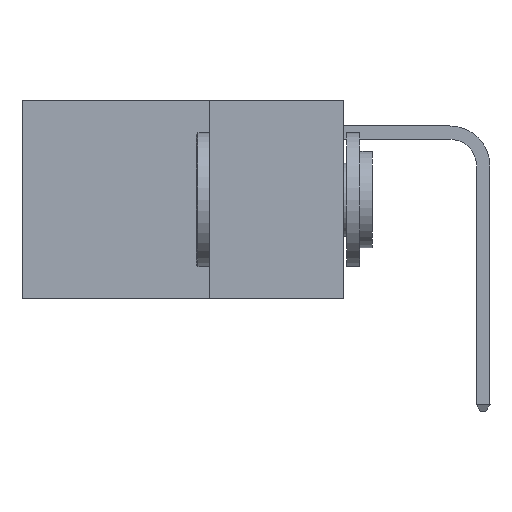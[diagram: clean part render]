
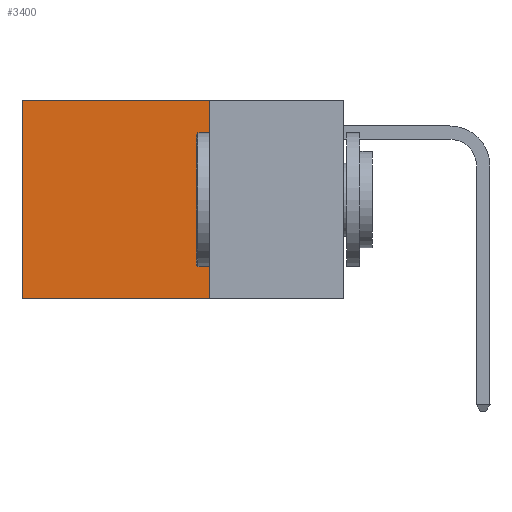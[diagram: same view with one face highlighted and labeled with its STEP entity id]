
A CAD part, left-side view. The second image highlights one B-rep face of the part: STEP entity #3400.
In plain terms, the highlighted planar face has unit normal (-1, 0, 0).
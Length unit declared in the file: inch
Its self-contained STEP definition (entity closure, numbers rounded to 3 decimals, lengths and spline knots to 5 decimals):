
#587 = CARTESIAN_POINT ( 'NONE',  ( 0.2625, 0.25, 0. ) ) ;
#814 = LINE ( 'NONE', #587, #7841 ) ;
#896 = LINE ( 'NONE', #6472, #7917 ) ;
#899 = CARTESIAN_POINT ( 'NONE',  ( 0.2625, 0.25, -0.37 ) ) ;
#993 = ORIENTED_EDGE ( 'NONE', *, *, #5014, .F. ) ;
#1522 = CARTESIAN_POINT ( 'NONE',  ( 0.2625, 0.25, 0. ) ) ;
#1548 = PLANE ( 'NONE',  #7059 ) ;
#1744 = VERTEX_POINT ( 'NONE', #6488 ) ;
#1950 = DIRECTION ( 'NONE',  ( 0., 0., -1. ) ) ;
#2151 = EDGE_LOOP ( 'NONE', ( #8183, #2232, #993, #2577 ) ) ;
#2232 = ORIENTED_EDGE ( 'NONE', *, *, #7408, .F. ) ;
#2319 = DIRECTION ( 'NONE',  ( 0., 1., 0. ) ) ;
#2573 = DIRECTION ( 'NONE',  ( 0., 0., -1. ) ) ;
#2577 = ORIENTED_EDGE ( 'NONE', *, *, #8396, .T. ) ;
#2618 = DIRECTION ( 'NONE',  ( 0., 1., 0. ) ) ;
#2760 = DIRECTION ( 'NONE',  ( 1., 0., 0. ) ) ;
#3400 = ADVANCED_FACE ( 'NONE', ( #5970 ), #1548, .F. ) ;
#4214 = VECTOR ( 'NONE', #2618, 39.37008 ) ;
#4866 = DIRECTION ( 'NONE',  ( 0., 0., -1. ) ) ;
#4922 = EDGE_CURVE ( 'NONE', #8659, #1744, #5209, .T. ) ;
#5014 = EDGE_CURVE ( 'NONE', #8641, #7359, #814, .T. ) ;
#5209 = LINE ( 'NONE', #5439, #6949 ) ;
#5410 = CARTESIAN_POINT ( 'NONE',  ( 0.2625, 0.25, 0. ) ) ;
#5439 = CARTESIAN_POINT ( 'NONE',  ( 0.2625, 0.6, 0. ) ) ;
#5683 = CARTESIAN_POINT ( 'NONE',  ( 0.2625, 0.25, 0. ) ) ;
#5970 = FACE_OUTER_BOUND ( 'NONE', #2151, .T. ) ;
#5984 = LINE ( 'NONE', #5410, #4214 ) ;
#6472 = CARTESIAN_POINT ( 'NONE',  ( 0.2625, 0.25, -0.37 ) ) ;
#6488 = CARTESIAN_POINT ( 'NONE',  ( 0.2625, 0.6, -0.37 ) ) ;
#6949 = VECTOR ( 'NONE', #1950, 39.37008 ) ;
#7059 = AXIS2_PLACEMENT_3D ( 'NONE', #1522, #2760, #2573 ) ;
#7359 = VERTEX_POINT ( 'NONE', #899 ) ;
#7408 = EDGE_CURVE ( 'NONE', #7359, #1744, #896, .T. ) ;
#7841 = VECTOR ( 'NONE', #4866, 39.37008 ) ;
#7917 = VECTOR ( 'NONE', #2319, 39.37008 ) ;
#8183 = ORIENTED_EDGE ( 'NONE', *, *, #4922, .T. ) ;
#8276 = CARTESIAN_POINT ( 'NONE',  ( 0.2625, 0.6, 0. ) ) ;
#8396 = EDGE_CURVE ( 'NONE', #8641, #8659, #5984, .T. ) ;
#8641 = VERTEX_POINT ( 'NONE', #5683 ) ;
#8659 = VERTEX_POINT ( 'NONE', #8276 ) ;
